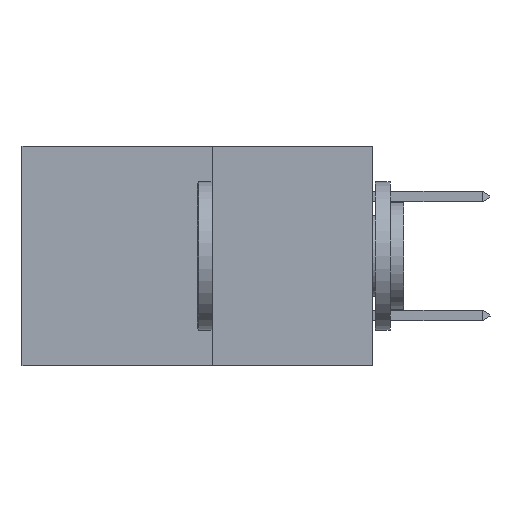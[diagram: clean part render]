
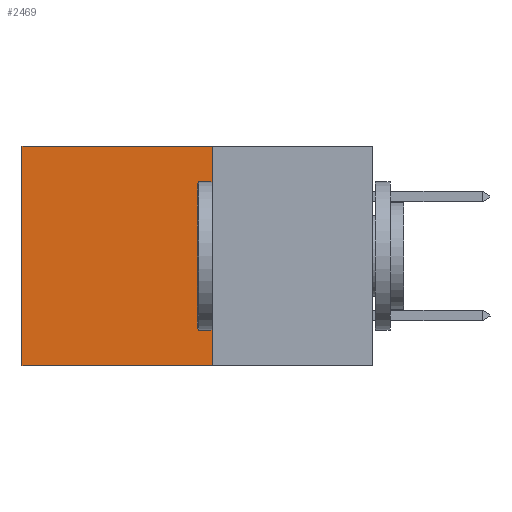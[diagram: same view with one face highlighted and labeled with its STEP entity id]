
A CAD part, left-side view. The second image highlights one B-rep face of the part: STEP entity #2469.
In plain terms, the highlighted planar face has unit normal (-1, 0, 0).
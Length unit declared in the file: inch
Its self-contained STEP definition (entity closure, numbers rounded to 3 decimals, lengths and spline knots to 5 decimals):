
#1558 = AXIS2_PLACEMENT_3D ( 'NONE', #8747, #6209, #6923 ) ;
#2172 = VECTOR ( 'NONE', #5294, 39.37008 ) ;
#2469 = ADVANCED_FACE ( 'NONE', ( #11239 ), #11750, .F. ) ;
#2473 = VERTEX_POINT ( 'NONE', #4821 ) ;
#2552 = VERTEX_POINT ( 'NONE', #5228 ) ;
#3897 = VERTEX_POINT ( 'NONE', #5957 ) ;
#4273 = VECTOR ( 'NONE', #10503, 39.37008 ) ;
#4533 = VECTOR ( 'NONE', #6023, 39.37008 ) ;
#4821 = CARTESIAN_POINT ( 'NONE',  ( 0.277, 0.59, -0.37 ) ) ;
#5228 = CARTESIAN_POINT ( 'NONE',  ( 0.277, 0.59, 0. ) ) ;
#5294 = DIRECTION ( 'NONE',  ( 0., 1., 0. ) ) ;
#5337 = CARTESIAN_POINT ( 'NONE',  ( 0.277, 0.27, 0. ) ) ;
#5957 = CARTESIAN_POINT ( 'NONE',  ( 0.277, 0.27, -0.37 ) ) ;
#6023 = DIRECTION ( 'NONE',  ( 0., 0., -1. ) ) ;
#6209 = DIRECTION ( 'NONE',  ( 1., 0., 0. ) ) ;
#6365 = ORIENTED_EDGE ( 'NONE', *, *, #10915, .T. ) ;
#6386 = EDGE_CURVE ( 'NONE', #3897, #2473, #12070, .T. ) ;
#6416 = LINE ( 'NONE', #11924, #11244 ) ;
#6511 = ORIENTED_EDGE ( 'NONE', *, *, #10290, .F. ) ;
#6714 = ORIENTED_EDGE ( 'NONE', *, *, #6386, .F. ) ;
#6923 = DIRECTION ( 'NONE',  ( 0., 0., -1. ) ) ;
#7301 = EDGE_LOOP ( 'NONE', ( #6365, #6714, #6511, #10992 ) ) ;
#7482 = LINE ( 'NONE', #5337, #2172 ) ;
#8042 = VERTEX_POINT ( 'NONE', #9088 ) ;
#8747 = CARTESIAN_POINT ( 'NONE',  ( 0.277, 0.27, -0.37 ) ) ;
#9037 = DIRECTION ( 'NONE',  ( 0., 0., -1. ) ) ;
#9088 = CARTESIAN_POINT ( 'NONE',  ( 0.277, 0.27, 0. ) ) ;
#9859 = CARTESIAN_POINT ( 'NONE',  ( 0.277, 0.59, -0.37 ) ) ;
#10018 = LINE ( 'NONE', #9859, #4533 ) ;
#10290 = EDGE_CURVE ( 'NONE', #8042, #3897, #6416, .T. ) ;
#10448 = EDGE_CURVE ( 'NONE', #8042, #2552, #7482, .T. ) ;
#10503 = DIRECTION ( 'NONE',  ( 0., 1., 0. ) ) ;
#10699 = CARTESIAN_POINT ( 'NONE',  ( 0.277, 0.27, -0.37 ) ) ;
#10915 = EDGE_CURVE ( 'NONE', #2552, #2473, #10018, .T. ) ;
#10992 = ORIENTED_EDGE ( 'NONE', *, *, #10448, .T. ) ;
#11239 = FACE_OUTER_BOUND ( 'NONE', #7301, .T. ) ;
#11244 = VECTOR ( 'NONE', #9037, 39.37008 ) ;
#11750 = PLANE ( 'NONE',  #1558 ) ;
#11924 = CARTESIAN_POINT ( 'NONE',  ( 0.277, 0.27, -0.37 ) ) ;
#12070 = LINE ( 'NONE', #10699, #4273 ) ;
